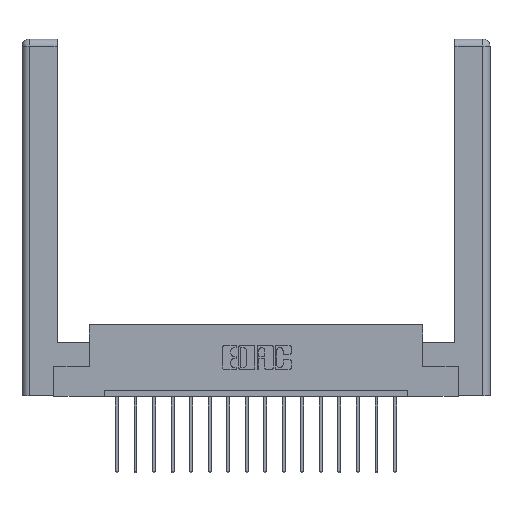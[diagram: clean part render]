
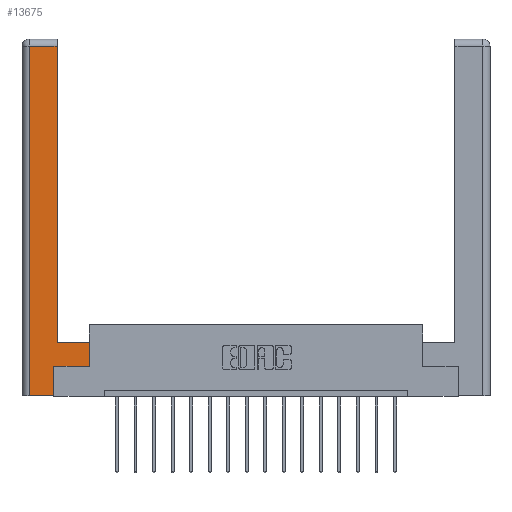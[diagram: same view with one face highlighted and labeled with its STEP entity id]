
A CAD part, top view. The second image highlights one B-rep face of the part: STEP entity #13675.
In plain terms, the highlighted planar face has unit normal (0, 0, 1).
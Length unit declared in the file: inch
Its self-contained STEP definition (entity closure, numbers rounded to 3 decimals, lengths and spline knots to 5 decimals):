
#550 = VECTOR ( 'NONE', #9594, 39.37008 ) ;
#682 = CARTESIAN_POINT ( 'NONE',  ( 0.265, 0.245, 0. ) ) ;
#811 = CARTESIAN_POINT ( 'NONE',  ( 0.565, 0.45, 0. ) ) ;
#1036 = DIRECTION ( 'NONE',  ( 0., -1., 0. ) ) ;
#1224 = CARTESIAN_POINT ( 'NONE',  ( 0.295, 0.45, 0. ) ) ;
#1547 = VECTOR ( 'NONE', #1036, 39.37008 ) ;
#1548 = ORIENTED_EDGE ( 'NONE', *, *, #11279, .T. ) ;
#1731 = LINE ( 'NONE', #6565, #11513 ) ;
#2399 = CARTESIAN_POINT ( 'NONE',  ( 0.565, 0.245, 0. ) ) ;
#2937 = VERTEX_POINT ( 'NONE', #2399 ) ;
#3175 = ORIENTED_EDGE ( 'NONE', *, *, #6098, .T. ) ;
#3213 = EDGE_CURVE ( 'NONE', #14170, #4120, #16826, .T. ) ;
#3236 = VERTEX_POINT ( 'NONE', #13031 ) ;
#3292 = CARTESIAN_POINT ( 'NONE',  ( 0.0615, 0., 0. ) ) ;
#4015 = LINE ( 'NONE', #9296, #12705 ) ;
#4120 = VERTEX_POINT ( 'NONE', #7888 ) ;
#4295 = DIRECTION ( 'NONE',  ( 0., 1., 0. ) ) ;
#4437 = VERTEX_POINT ( 'NONE', #682 ) ;
#4770 = LINE ( 'NONE', #9689, #5854 ) ;
#5709 = ORIENTED_EDGE ( 'NONE', *, *, #8516, .T. ) ;
#5823 = CARTESIAN_POINT ( 'NONE',  ( 0.0615, 0., 0. ) ) ;
#5854 = VECTOR ( 'NONE', #4295, 39.37008 ) ;
#6083 = DIRECTION ( 'NONE',  ( 1., 0., 0. ) ) ;
#6098 = EDGE_CURVE ( 'NONE', #3236, #4437, #4770, .T. ) ;
#6565 = CARTESIAN_POINT ( 'NONE',  ( 0.295, 0.45, 0. ) ) ;
#6629 = ORIENTED_EDGE ( 'NONE', *, *, #15405, .T. ) ;
#7185 = CARTESIAN_POINT ( 'NONE',  ( 0.565, 0.245, 0. ) ) ;
#7450 = LINE ( 'NONE', #5823, #1547 ) ;
#7763 = LINE ( 'NONE', #14876, #550 ) ;
#7784 = EDGE_CURVE ( 'NONE', #7799, #3236, #17206, .T. ) ;
#7799 = VERTEX_POINT ( 'NONE', #3292 ) ;
#7829 = FACE_OUTER_BOUND ( 'NONE', #12543, .T. ) ;
#7888 = CARTESIAN_POINT ( 'NONE',  ( 0.295, 2.94, 0. ) ) ;
#8131 = PLANE ( 'NONE',  #14123 ) ;
#8255 = ORIENTED_EDGE ( 'NONE', *, *, #9936, .T. ) ;
#8448 = DIRECTION ( 'NONE',  ( 1., 0., 0. ) ) ;
#8516 = EDGE_CURVE ( 'NONE', #4120, #13362, #4015, .T. ) ;
#9157 = CARTESIAN_POINT ( 'NONE',  ( 0.295, 3., 0. ) ) ;
#9295 = ORIENTED_EDGE ( 'NONE', *, *, #12358, .T. ) ;
#9296 = CARTESIAN_POINT ( 'NONE',  ( 0.0615, 2.94, 0. ) ) ;
#9533 = DIRECTION ( 'NONE',  ( -1., 0., 0. ) ) ;
#9594 = DIRECTION ( 'NONE',  ( 0., 1., 0. ) ) ;
#9689 = CARTESIAN_POINT ( 'NONE',  ( 0.265, 0.245, 0. ) ) ;
#9936 = EDGE_CURVE ( 'NONE', #4437, #2937, #14769, .T. ) ;
#10583 = VECTOR ( 'NONE', #14565, 39.37008 ) ;
#11129 = VECTOR ( 'NONE', #8448, 39.37008 ) ;
#11279 = EDGE_CURVE ( 'NONE', #13294, #14170, #1731, .T. ) ;
#11513 = VECTOR ( 'NONE', #12123, 39.37008 ) ;
#11891 = DIRECTION ( 'NONE',  ( -1., 0., 0. ) ) ;
#12123 = DIRECTION ( 'NONE',  ( -1., 0., 0. ) ) ;
#12357 = CARTESIAN_POINT ( 'NONE',  ( 0., 0., 0. ) ) ;
#12358 = EDGE_CURVE ( 'NONE', #13362, #7799, #7450, .T. ) ;
#12543 = EDGE_LOOP ( 'NONE', ( #12972, #5709, #9295, #15017, #3175, #8255, #6629, #1548 ) ) ;
#12705 = VECTOR ( 'NONE', #11891, 39.37008 ) ;
#12972 = ORIENTED_EDGE ( 'NONE', *, *, #3213, .T. ) ;
#13031 = CARTESIAN_POINT ( 'NONE',  ( 0.265, 0., 0. ) ) ;
#13294 = VERTEX_POINT ( 'NONE', #811 ) ;
#13362 = VERTEX_POINT ( 'NONE', #15085 ) ;
#13675 = ADVANCED_FACE ( 'NONE', ( #7829 ), #8131, .F. ) ;
#14123 = AXIS2_PLACEMENT_3D ( 'NONE', #12357, #17806, #9533 ) ;
#14170 = VERTEX_POINT ( 'NONE', #1224 ) ;
#14565 = DIRECTION ( 'NONE',  ( 0., 1., 0. ) ) ;
#14769 = LINE ( 'NONE', #7185, #11129 ) ;
#14876 = CARTESIAN_POINT ( 'NONE',  ( 0.565, 0.45, 0. ) ) ;
#15017 = ORIENTED_EDGE ( 'NONE', *, *, #7784, .T. ) ;
#15085 = CARTESIAN_POINT ( 'NONE',  ( 0.0615, 2.94, 0. ) ) ;
#15405 = EDGE_CURVE ( 'NONE', #2937, #13294, #7763, .T. ) ;
#16135 = VECTOR ( 'NONE', #6083, 39.37008 ) ;
#16826 = LINE ( 'NONE', #9157, #10583 ) ;
#16999 = CARTESIAN_POINT ( 'NONE',  ( 0.265, 0., 0. ) ) ;
#17206 = LINE ( 'NONE', #16999, #16135 ) ;
#17806 = DIRECTION ( 'NONE',  ( 0., 0., -1. ) ) ;
